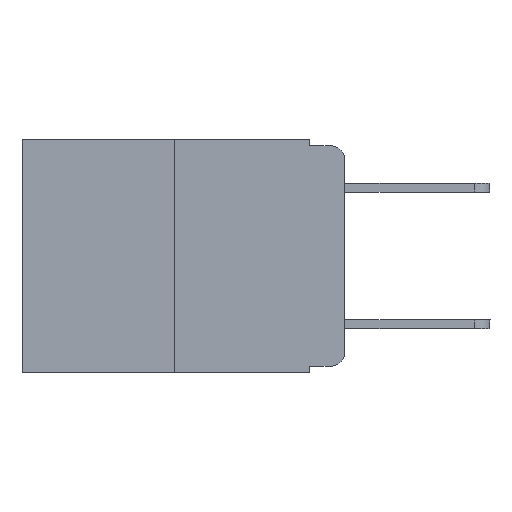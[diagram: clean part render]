
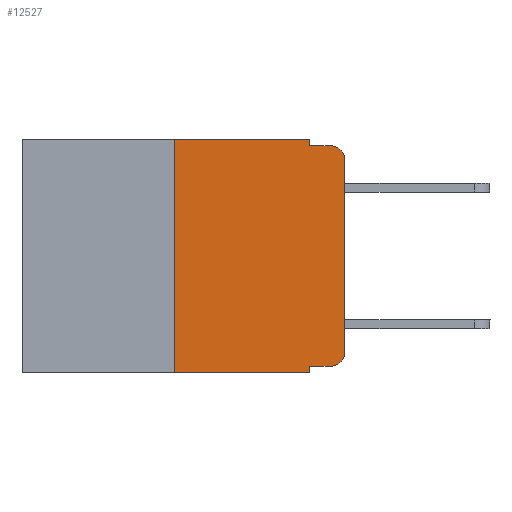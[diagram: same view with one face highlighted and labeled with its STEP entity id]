
A CAD part, left-side view. The second image highlights one B-rep face of the part: STEP entity #12527.
In plain terms, the highlighted planar face has unit normal (-1, 0, 0).
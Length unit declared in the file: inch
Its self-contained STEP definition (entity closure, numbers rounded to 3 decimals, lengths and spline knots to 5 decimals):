
#4 = DIRECTION ( 'NONE',  ( 0., 0., -1. ) ) ;
#362 = CARTESIAN_POINT ( 'NONE',  ( 0., 0.25, -0.343 ) ) ;
#409 = CIRCLE ( 'NONE', #10845, 0.02 ) ;
#557 = EDGE_CURVE ( 'NONE', #12574, #11112, #409, .T. ) ;
#636 = VECTOR ( 'NONE', #12784, 39.37008 ) ;
#660 = CARTESIAN_POINT ( 'NONE',  ( 0., 0.051, -0.333 ) ) ;
#785 = VERTEX_POINT ( 'NONE', #12814 ) ;
#872 = DIRECTION ( 'NONE',  ( 0., 0., 1. ) ) ;
#1390 = DIRECTION ( 'NONE',  ( 0., -1., 0. ) ) ;
#1432 = CARTESIAN_POINT ( 'NONE',  ( 0., 0.25, 0. ) ) ;
#1583 = ORIENTED_EDGE ( 'NONE', *, *, #5705, .F. ) ;
#1621 = VECTOR ( 'NONE', #6746, 39.37008 ) ;
#1630 = LINE ( 'NONE', #7973, #12729 ) ;
#1675 = CARTESIAN_POINT ( 'NONE',  ( 0., 0.473, 0. ) ) ;
#1770 = PLANE ( 'NONE',  #7603 ) ;
#1918 = CARTESIAN_POINT ( 'NONE',  ( 0., 0.051, -0.333 ) ) ;
#2304 = CARTESIAN_POINT ( 'NONE',  ( 0., 0.25, 0. ) ) ;
#2567 = ORIENTED_EDGE ( 'NONE', *, *, #5901, .F. ) ;
#2782 = DIRECTION ( 'NONE',  ( 1., 0., 0. ) ) ;
#2889 = VECTOR ( 'NONE', #2994, 39.37008 ) ;
#2914 = EDGE_CURVE ( 'NONE', #8978, #8544, #3766, .T. ) ;
#2962 = ORIENTED_EDGE ( 'NONE', *, *, #2914, .T. ) ;
#2994 = DIRECTION ( 'NONE',  ( 0., -1., 0. ) ) ;
#3039 = EDGE_CURVE ( 'NONE', #9940, #785, #4960, .T. ) ;
#3340 = VECTOR ( 'NONE', #872, 39.37008 ) ;
#3494 = DIRECTION ( 'NONE',  ( 0., 0., 1. ) ) ;
#3534 = LINE ( 'NONE', #660, #636 ) ;
#3703 = FACE_OUTER_BOUND ( 'NONE', #5813, .T. ) ;
#3766 = LINE ( 'NONE', #4827, #5843 ) ;
#3982 = DIRECTION ( 'NONE',  ( 0., 0., -1. ) ) ;
#4351 = CARTESIAN_POINT ( 'NONE',  ( 0., 0., -0.313 ) ) ;
#4704 = VECTOR ( 'NONE', #4, 39.37008 ) ;
#4715 = VERTEX_POINT ( 'NONE', #7229 ) ;
#4773 = ORIENTED_EDGE ( 'NONE', *, *, #557, .T. ) ;
#4777 = DIRECTION ( 'NONE',  ( 0., -1., 0. ) ) ;
#4827 = CARTESIAN_POINT ( 'NONE',  ( 0., 0.473, -0.343 ) ) ;
#4960 = LINE ( 'NONE', #9588, #2889 ) ;
#5018 = CARTESIAN_POINT ( 'NONE',  ( 0., 0.02, -0.03 ) ) ;
#5234 = EDGE_CURVE ( 'NONE', #9231, #8544, #12894, .T. ) ;
#5418 = EDGE_CURVE ( 'NONE', #12748, #12574, #13589, .T. ) ;
#5520 = DIRECTION ( 'NONE',  ( 0., 0., -1. ) ) ;
#5696 = CARTESIAN_POINT ( 'NONE',  ( 0., 0.051, 0. ) ) ;
#5705 = EDGE_CURVE ( 'NONE', #785, #12590, #9871, .T. ) ;
#5813 = EDGE_LOOP ( 'NONE', ( #9469, #4773, #12068, #1583, #5966, #2567, #2962, #9491, #7359, #13767 ) ) ;
#5843 = VECTOR ( 'NONE', #4777, 39.37008 ) ;
#5901 = EDGE_CURVE ( 'NONE', #8978, #9940, #11659, .T. ) ;
#5966 = ORIENTED_EDGE ( 'NONE', *, *, #3039, .F. ) ;
#6066 = CARTESIAN_POINT ( 'NONE',  ( 0., 0., -0.03 ) ) ;
#6250 = CARTESIAN_POINT ( 'NONE',  ( 0., 0.051, -0.01 ) ) ;
#6746 = DIRECTION ( 'NONE',  ( 0., 0., -1. ) ) ;
#7122 = AXIS2_PLACEMENT_3D ( 'NONE', #8690, #7778, #5520 ) ;
#7229 = CARTESIAN_POINT ( 'NONE',  ( 0., 0.02, -0.333 ) ) ;
#7359 = ORIENTED_EDGE ( 'NONE', *, *, #11872, .T. ) ;
#7603 = AXIS2_PLACEMENT_3D ( 'NONE', #1675, #2782, #3982 ) ;
#7778 = DIRECTION ( 'NONE',  ( -1., 0., 0. ) ) ;
#7973 = CARTESIAN_POINT ( 'NONE',  ( 0., 0.051, -0.01 ) ) ;
#8240 = CARTESIAN_POINT ( 'NONE',  ( 0., 0., 0. ) ) ;
#8544 = VERTEX_POINT ( 'NONE', #10548 ) ;
#8690 = CARTESIAN_POINT ( 'NONE',  ( 0., 0.02, -0.313 ) ) ;
#8840 = CARTESIAN_POINT ( 'NONE',  ( 0., 0.051, 0. ) ) ;
#8978 = VERTEX_POINT ( 'NONE', #362 ) ;
#9231 = VERTEX_POINT ( 'NONE', #1918 ) ;
#9469 = ORIENTED_EDGE ( 'NONE', *, *, #5418, .T. ) ;
#9491 = ORIENTED_EDGE ( 'NONE', *, *, #5234, .F. ) ;
#9588 = CARTESIAN_POINT ( 'NONE',  ( 0., 0.473, 0. ) ) ;
#9871 = LINE ( 'NONE', #8840, #4704 ) ;
#9936 = EDGE_CURVE ( 'NONE', #4715, #12748, #11935, .T. ) ;
#9940 = VERTEX_POINT ( 'NONE', #2304 ) ;
#10548 = CARTESIAN_POINT ( 'NONE',  ( 0., 0.051, -0.343 ) ) ;
#10845 = AXIS2_PLACEMENT_3D ( 'NONE', #5018, #12793, #11540 ) ;
#11112 = VERTEX_POINT ( 'NONE', #14241 ) ;
#11540 = DIRECTION ( 'NONE',  ( 0., 0., -1. ) ) ;
#11659 = LINE ( 'NONE', #1432, #13575 ) ;
#11872 = EDGE_CURVE ( 'NONE', #9231, #4715, #3534, .T. ) ;
#11935 = CIRCLE ( 'NONE', #7122, 0.02 ) ;
#12068 = ORIENTED_EDGE ( 'NONE', *, *, #12909, .F. ) ;
#12527 = ADVANCED_FACE ( 'NONE', ( #3703 ), #1770, .F. ) ;
#12574 = VERTEX_POINT ( 'NONE', #6066 ) ;
#12590 = VERTEX_POINT ( 'NONE', #6250 ) ;
#12729 = VECTOR ( 'NONE', #1390, 39.37008 ) ;
#12748 = VERTEX_POINT ( 'NONE', #4351 ) ;
#12784 = DIRECTION ( 'NONE',  ( 0., -1., 0. ) ) ;
#12793 = DIRECTION ( 'NONE',  ( -1., 0., 0. ) ) ;
#12814 = CARTESIAN_POINT ( 'NONE',  ( 0., 0.051, 0. ) ) ;
#12894 = LINE ( 'NONE', #5696, #1621 ) ;
#12909 = EDGE_CURVE ( 'NONE', #12590, #11112, #1630, .T. ) ;
#13575 = VECTOR ( 'NONE', #3494, 39.37008 ) ;
#13589 = LINE ( 'NONE', #8240, #3340 ) ;
#13767 = ORIENTED_EDGE ( 'NONE', *, *, #9936, .T. ) ;
#14241 = CARTESIAN_POINT ( 'NONE',  ( 0., 0.02, -0.01 ) ) ;
